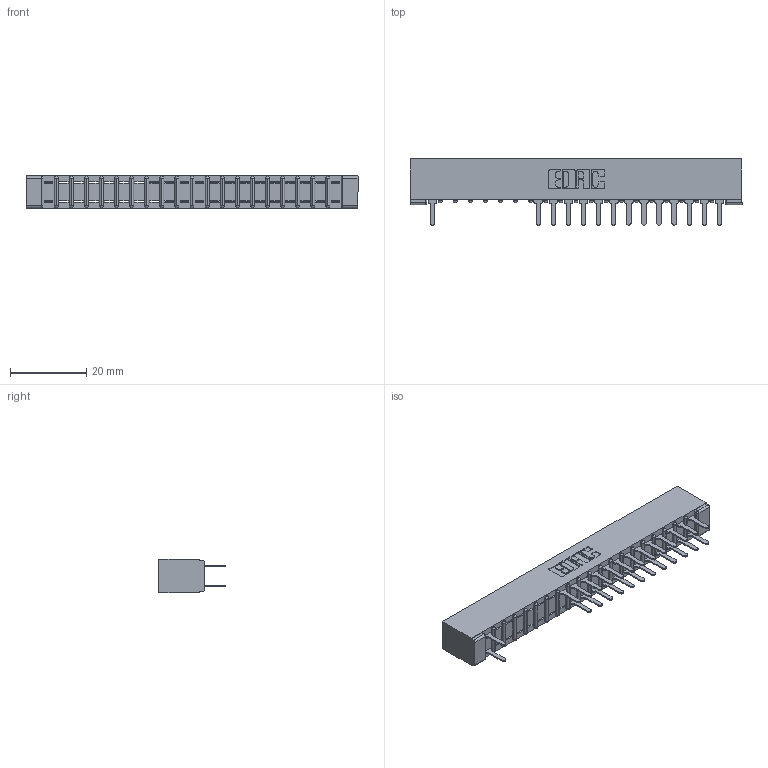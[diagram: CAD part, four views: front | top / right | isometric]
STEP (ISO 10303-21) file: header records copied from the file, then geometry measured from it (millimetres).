
FILE_DESCRIPTION (( 'STEP AP203' ), '1' );
FILE_NAME ('307-040-520-201.STEP', '2018-08-05T14:38:33', ( '' ), ( '' ), 'SwSTEP 2.0', 'SolidWorks 2016', '' );
FILE_SCHEMA (( 'CONFIG_CONTROL_DESIGN' ));
Length unit declared in the file: inch
Products named in the file (3): 307 Part_No Mounting Lugs; 307-290-001_520; 307-040-520-201
Assembly tree (28 placements, depth 2):
  307-040-520-201
    307 Part_No Mounting Lugs
    307-290-001_520  x27
Bounding box: 87.12 x 17.42 x 8.71 mm (x, y, z)
Volume: 5783.5 mm3; surface area: 9661.6 mm2
Topology: 28 solids, 28 shells, 1503 faces, 4225 edges, 2722 vertices
Faces by surface type: plane 981, cylinder 480, sphere 42
Entity records: 19772 total; most frequent: CARTESIAN_POINT 3291, ORIENTED_EDGE 3270, DIRECTION 3219, EDGE_CURVE 1635, VECTOR 1247, LINE 1247, VERTEX_POINT 1058, AXIS2_PLACEMENT_3D 986
